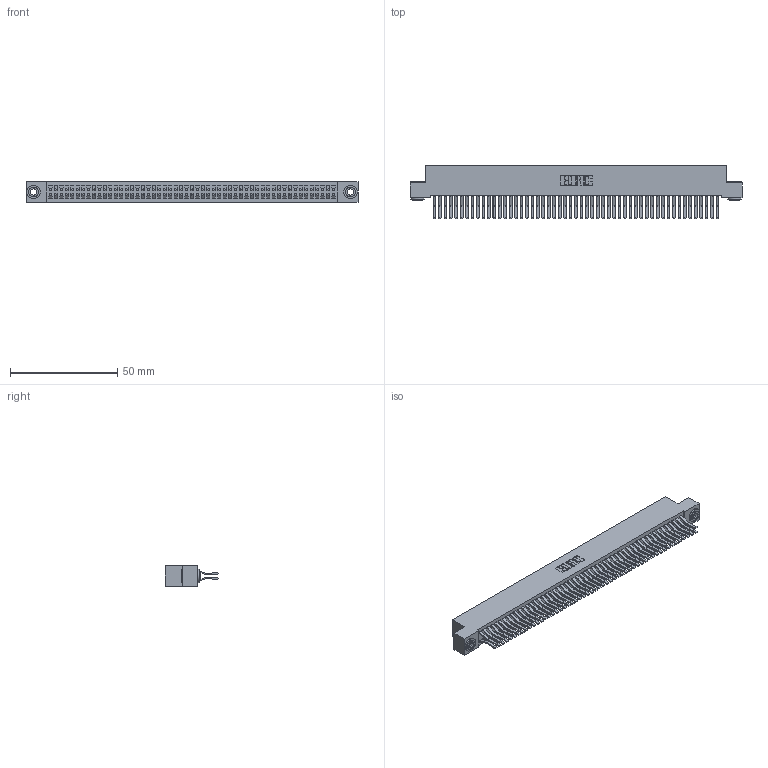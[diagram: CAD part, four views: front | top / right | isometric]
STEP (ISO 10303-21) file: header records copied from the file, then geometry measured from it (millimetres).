
FILE_DESCRIPTION (( 'STEP AP203' ), '1' );
FILE_NAME ('342-106-560-203.STEP', '2019-10-04T19:30:50', ( '' ), ( '' ), 'SwSTEP 2.0', 'SolidWorks 2016', '' );
FILE_SCHEMA (( 'CONFIG_CONTROL_DESIGN' ));
Length unit declared in the file: inch
Products named in the file (4): 342 Part_.156 TH; 345-292-001_560 Tail; 342-250-002_345-250-002-102; 342-106-560-203
Assembly tree (109 placements, depth 2):
  342-106-560-203
    342 Part_.156 TH
    345-292-001_560 Tail  x106
    342-250-002_345-250-002-102  x2
Bounding box: 154.94 x 24.78 x 9.4 mm (x, y, z)
Volume: 14692.1 mm3; surface area: 26069 mm2
Topology: 109 solids, 109 shells, 5872 faces, 17441 edges, 11482 vertices
Faces by surface type: plane 3892, cylinder 1972, cone 8
Entity records: 33280 total; most frequent: CARTESIAN_POINT 5477, ORIENTED_EDGE 5406, DIRECTION 4697, EDGE_CURVE 2703, LINE 2547, VECTOR 2547, VERTEX_POINT 1798, AXIS2_PLACEMENT_3D 1075
